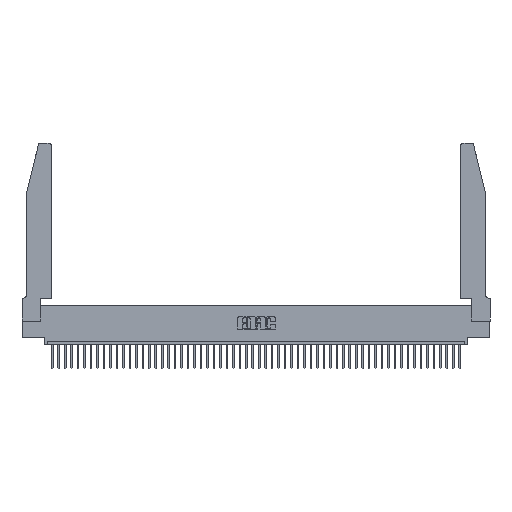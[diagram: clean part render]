
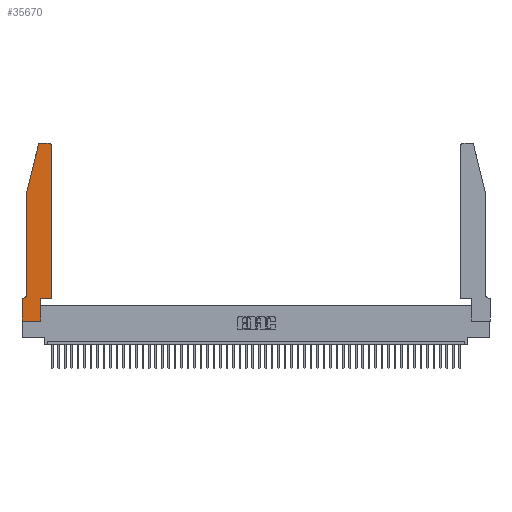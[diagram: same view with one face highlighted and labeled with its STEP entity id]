
A CAD part, top view. The second image highlights one B-rep face of the part: STEP entity #35670.
In plain terms, the highlighted planar face has unit normal (0, 0, 1).
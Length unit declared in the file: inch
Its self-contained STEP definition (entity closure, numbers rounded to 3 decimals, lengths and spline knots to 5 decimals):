
#377 = VECTOR ( 'NONE', #6063, 39.37008 ) ;
#442 = VERTEX_POINT ( 'NONE', #46112 ) ;
#886 = DIRECTION ( 'NONE',  ( -1., 0., 0. ) ) ;
#1024 = LINE ( 'NONE', #24592, #36820 ) ;
#1542 = DIRECTION ( 'NONE',  ( 1., 0., 0. ) ) ;
#2826 = CARTESIAN_POINT ( 'NONE',  ( 0.2865, 0., 0.37 ) ) ;
#3449 = VECTOR ( 'NONE', #886, 39.37008 ) ;
#3791 = CARTESIAN_POINT ( 'NONE',  ( 0.2865, 0.35, 0.37 ) ) ;
#3968 = ORIENTED_EDGE ( 'NONE', *, *, #48173, .T. ) ;
#3980 = CARTESIAN_POINT ( 'NONE',  ( 0.4505, 2.72, 0.37 ) ) ;
#4018 = VERTEX_POINT ( 'NONE', #4857 ) ;
#4459 = EDGE_CURVE ( 'NONE', #4018, #44024, #9153, .T. ) ;
#4857 = CARTESIAN_POINT ( 'NONE',  ( 0., 0.35, 0.37 ) ) ;
#4873 = DIRECTION ( 'NONE',  ( 0., -1., 0. ) ) ;
#5049 = CARTESIAN_POINT ( 'NONE',  ( 0.0755, 0.35, 0.37 ) ) ;
#5397 = DIRECTION ( 'NONE',  ( 1., 0., 0. ) ) ;
#5418 = CIRCLE ( 'NONE', #27611, 0.03 ) ;
#6063 = DIRECTION ( 'NONE',  ( -0.239, -0.971, 0. ) ) ;
#6480 = EDGE_LOOP ( 'NONE', ( #39313, #24898, #10403, #23533, #47323, #19569, #39560, #26907, #28335, #44920, #38873, #3968 ) ) ;
#6880 = VERTEX_POINT ( 'NONE', #2826 ) ;
#9050 = PLANE ( 'NONE',  #18370 ) ;
#9153 = LINE ( 'NONE', #47008, #47306 ) ;
#9614 = DIRECTION ( 'NONE',  ( -1., 0., 0. ) ) ;
#10403 = ORIENTED_EDGE ( 'NONE', *, *, #29768, .T. ) ;
#11112 = EDGE_CURVE ( 'NONE', #22924, #16494, #32630, .T. ) ;
#11320 = DIRECTION ( 'NONE',  ( 0., 0., 1. ) ) ;
#12640 = CARTESIAN_POINT ( 'NONE',  ( 0.284, 2.75, 0.37 ) ) ;
#13430 = DIRECTION ( 'NONE',  ( 1., 0., 0. ) ) ;
#13706 = LINE ( 'NONE', #44282, #3449 ) ;
#15071 = VECTOR ( 'NONE', #23953, 39.37008 ) ;
#15195 = DIRECTION ( 'NONE',  ( 1., 0., 0. ) ) ;
#15326 = EDGE_CURVE ( 'NONE', #41686, #442, #39085, .T. ) ;
#15720 = CARTESIAN_POINT ( 'NONE',  ( 0.2865, 0.35, 0.37 ) ) ;
#16494 = VERTEX_POINT ( 'NONE', #19971 ) ;
#18370 = AXIS2_PLACEMENT_3D ( 'NONE', #23848, #11320, #13430 ) ;
#18702 = CARTESIAN_POINT ( 'NONE',  ( 0.0755, 2., 0.37 ) ) ;
#18916 = CARTESIAN_POINT ( 'NONE',  ( 0.0755, 2., 0.37 ) ) ;
#19027 = AXIS2_PLACEMENT_3D ( 'NONE', #29418, #33288, #9614 ) ;
#19314 = VERTEX_POINT ( 'NONE', #3791 ) ;
#19552 = VECTOR ( 'NONE', #29922, 39.37008 ) ;
#19569 = ORIENTED_EDGE ( 'NONE', *, *, #39047, .T. ) ;
#19971 = CARTESIAN_POINT ( 'NONE',  ( 0.0055, 0.35, 0.37 ) ) ;
#20454 = VERTEX_POINT ( 'NONE', #36526 ) ;
#20753 = VECTOR ( 'NONE', #36359, 39.37008 ) ;
#20905 = CARTESIAN_POINT ( 'NONE',  ( 0.4505, 0.35, 0.37 ) ) ;
#20955 = EDGE_CURVE ( 'NONE', #20454, #24856, #30517, .T. ) ;
#22768 = DIRECTION ( 'NONE',  ( 0., 0., 1. ) ) ;
#22924 = VERTEX_POINT ( 'NONE', #24217 ) ;
#23533 = ORIENTED_EDGE ( 'NONE', *, *, #33259, .T. ) ;
#23748 = FACE_OUTER_BOUND ( 'NONE', #6480, .T. ) ;
#23848 = CARTESIAN_POINT ( 'NONE',  ( 0., 0.35, 0.37 ) ) ;
#23953 = DIRECTION ( 'NONE',  ( -1., 0., 0. ) ) ;
#24217 = CARTESIAN_POINT ( 'NONE',  ( 0.0755, 0.42, 0.37 ) ) ;
#24592 = CARTESIAN_POINT ( 'NONE',  ( 0., 0., 0.37 ) ) ;
#24856 = VERTEX_POINT ( 'NONE', #3980 ) ;
#24898 = ORIENTED_EDGE ( 'NONE', *, *, #15326, .T. ) ;
#26509 = CARTESIAN_POINT ( 'NONE',  ( 0.4205, 2.72, 0.37 ) ) ;
#26612 = AXIS2_PLACEMENT_3D ( 'NONE', #33089, #49032, #41274 ) ;
#26907 = ORIENTED_EDGE ( 'NONE', *, *, #29098, .T. ) ;
#27611 = AXIS2_PLACEMENT_3D ( 'NONE', #26509, #22768, #15195 ) ;
#28335 = ORIENTED_EDGE ( 'NONE', *, *, #42979, .T. ) ;
#29098 = EDGE_CURVE ( 'NONE', #44024, #6880, #1024, .T. ) ;
#29206 = CARTESIAN_POINT ( 'NONE',  ( 0.0755, 2., 0.37 ) ) ;
#29418 = CARTESIAN_POINT ( 'NONE',  ( 0.0055, 0.42, 0.37 ) ) ;
#29768 = EDGE_CURVE ( 'NONE', #442, #43434, #48210, .T. ) ;
#29922 = DIRECTION ( 'NONE',  ( 0., -1., 0. ) ) ;
#30517 = LINE ( 'NONE', #43852, #20753 ) ;
#31885 = EDGE_CURVE ( 'NONE', #19314, #20454, #43842, .T. ) ;
#32630 = CIRCLE ( 'NONE', #19027, 0.07 ) ;
#33089 = CARTESIAN_POINT ( 'NONE',  ( 0.284, 2.72, 0.37 ) ) ;
#33259 = EDGE_CURVE ( 'NONE', #43434, #22924, #33694, .T. ) ;
#33288 = DIRECTION ( 'NONE',  ( 0., 0., -1. ) ) ;
#33694 = LINE ( 'NONE', #18916, #19552 ) ;
#34837 = DIRECTION ( 'NONE',  ( 0., 1., 0. ) ) ;
#35670 = ADVANCED_FACE ( 'NONE', ( #23748 ), #9050, .T. ) ;
#36359 = DIRECTION ( 'NONE',  ( 0., 1., 0. ) ) ;
#36526 = CARTESIAN_POINT ( 'NONE',  ( 0.4505, 0.35, 0.37 ) ) ;
#36820 = VECTOR ( 'NONE', #1542, 39.37008 ) ;
#37055 = VECTOR ( 'NONE', #34837, 39.37008 ) ;
#38873 = ORIENTED_EDGE ( 'NONE', *, *, #20955, .T. ) ;
#39047 = EDGE_CURVE ( 'NONE', #16494, #4018, #49559, .T. ) ;
#39085 = CIRCLE ( 'NONE', #26612, 0.03 ) ;
#39313 = ORIENTED_EDGE ( 'NONE', *, *, #41226, .T. ) ;
#39560 = ORIENTED_EDGE ( 'NONE', *, *, #4459, .T. ) ;
#40107 = LINE ( 'NONE', #15720, #37055 ) ;
#41226 = EDGE_CURVE ( 'NONE', #46785, #41686, #13706, .T. ) ;
#41274 = DIRECTION ( 'NONE',  ( 1., 0., 0. ) ) ;
#41686 = VERTEX_POINT ( 'NONE', #12640 ) ;
#42979 = EDGE_CURVE ( 'NONE', #6880, #19314, #40107, .T. ) ;
#43434 = VERTEX_POINT ( 'NONE', #18702 ) ;
#43842 = LINE ( 'NONE', #20905, #47445 ) ;
#43852 = CARTESIAN_POINT ( 'NONE',  ( 0.4505, 0.35, 0.37 ) ) ;
#44024 = VERTEX_POINT ( 'NONE', #49598 ) ;
#44282 = CARTESIAN_POINT ( 'NONE',  ( 0.2605, 2.75, 0.37 ) ) ;
#44920 = ORIENTED_EDGE ( 'NONE', *, *, #31885, .T. ) ;
#46112 = CARTESIAN_POINT ( 'NONE',  ( 0.25487, 2.72718, 0.37 ) ) ;
#46785 = VERTEX_POINT ( 'NONE', #48026 ) ;
#47008 = CARTESIAN_POINT ( 'NONE',  ( 0., 0., 0.37 ) ) ;
#47306 = VECTOR ( 'NONE', #4873, 39.37008 ) ;
#47323 = ORIENTED_EDGE ( 'NONE', *, *, #11112, .T. ) ;
#47445 = VECTOR ( 'NONE', #5397, 39.37008 ) ;
#48026 = CARTESIAN_POINT ( 'NONE',  ( 0.4205, 2.75, 0.37 ) ) ;
#48173 = EDGE_CURVE ( 'NONE', #24856, #46785, #5418, .T. ) ;
#48210 = LINE ( 'NONE', #29206, #377 ) ;
#49032 = DIRECTION ( 'NONE',  ( 0., 0., 1. ) ) ;
#49559 = LINE ( 'NONE', #5049, #15071 ) ;
#49598 = CARTESIAN_POINT ( 'NONE',  ( 0., 0., 0.37 ) ) ;
